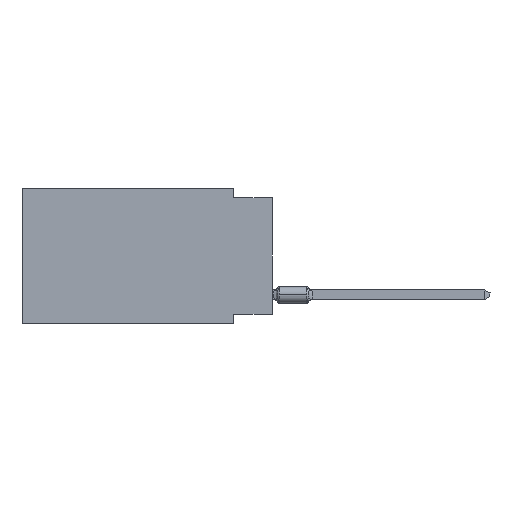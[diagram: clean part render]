
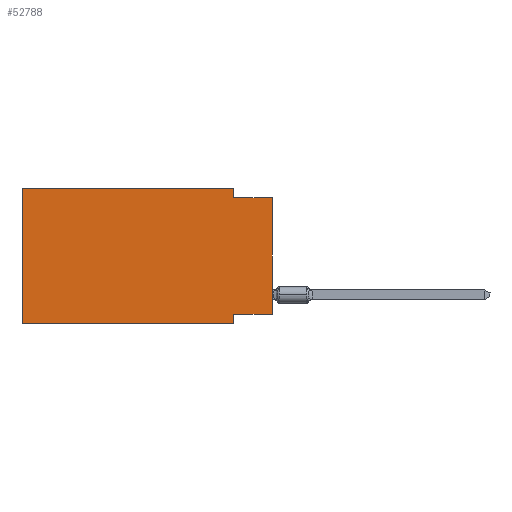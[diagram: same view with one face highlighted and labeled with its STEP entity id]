
A CAD part, left-side view. The second image highlights one B-rep face of the part: STEP entity #52788.
In plain terms, the highlighted planar face has unit normal (-1, 0, 0).
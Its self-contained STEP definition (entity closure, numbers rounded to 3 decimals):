
#1383 = DIRECTION ( 'NONE',  ( 0., -1., 0. ) ) ;
#1533 = ORIENTED_EDGE ( 'NONE', *, *, #18060, .F. ) ;
#2192 = VECTOR ( 'NONE', #11639, 1000. ) ;
#2943 = DIRECTION ( 'NONE',  ( 1., 0., 0. ) ) ;
#3807 = VECTOR ( 'NONE', #10989, 1000. ) ;
#5880 = CARTESIAN_POINT ( 'NONE',  ( 0., 2.54, 0. ) ) ;
#6173 = CARTESIAN_POINT ( 'NONE',  ( 0., 16.383, 0. ) ) ;
#8755 = LINE ( 'NONE', #69886, #24046 ) ;
#9847 = DIRECTION ( 'NONE',  ( 0., -1., 0. ) ) ;
#10810 = DIRECTION ( 'NONE',  ( 0., 0., -1. ) ) ;
#10989 = DIRECTION ( 'NONE',  ( 0., 1., 0. ) ) ;
#11277 = EDGE_CURVE ( 'NONE', #36131, #18457, #34651, .T. ) ;
#11639 = DIRECTION ( 'NONE',  ( 0., -1., 0. ) ) ;
#15030 = LINE ( 'NONE', #37718, #3807 ) ;
#15387 = EDGE_CURVE ( 'NONE', #43830, #36131, #8755, .T. ) ;
#15999 = VERTEX_POINT ( 'NONE', #23477 ) ;
#18060 = EDGE_CURVE ( 'NONE', #28030, #43830, #68750, .T. ) ;
#18457 = VERTEX_POINT ( 'NONE', #68885 ) ;
#18675 = EDGE_LOOP ( 'NONE', ( #70480, #69194, #62067, #1533, #72188, #52999, #63811, #28045 ) ) ;
#19309 = VECTOR ( 'NONE', #9847, 1000. ) ;
#19745 = CARTESIAN_POINT ( 'NONE',  ( 0., 16.383, 0. ) ) ;
#20841 = VERTEX_POINT ( 'NONE', #34207 ) ;
#22813 = EDGE_CURVE ( 'NONE', #15999, #20841, #15030, .T. ) ;
#23095 = CARTESIAN_POINT ( 'NONE',  ( 0., 0., 0. ) ) ;
#23446 = LINE ( 'NONE', #23095, #54664 ) ;
#23477 = CARTESIAN_POINT ( 'NONE',  ( 0., 0., -8.255 ) ) ;
#24046 = VECTOR ( 'NONE', #24820, 1000. ) ;
#24353 = VECTOR ( 'NONE', #10810, 1000. ) ;
#24820 = DIRECTION ( 'NONE',  ( 0., 0., -1. ) ) ;
#24863 = DIRECTION ( 'NONE',  ( 0., 0., -1. ) ) ;
#28030 = VERTEX_POINT ( 'NONE', #56153 ) ;
#28045 = ORIENTED_EDGE ( 'NONE', *, *, #22813, .F. ) ;
#28693 = CARTESIAN_POINT ( 'NONE',  ( 0., 2.54, -0.635 ) ) ;
#31381 = CARTESIAN_POINT ( 'NONE',  ( 0., 16.383, 0. ) ) ;
#32398 = CARTESIAN_POINT ( 'NONE',  ( 0., 2.54, -8.89 ) ) ;
#34207 = CARTESIAN_POINT ( 'NONE',  ( 0., 2.54, -8.255 ) ) ;
#34354 = VECTOR ( 'NONE', #52305, 1000. ) ;
#34651 = LINE ( 'NONE', #39442, #43496 ) ;
#36131 = VERTEX_POINT ( 'NONE', #28693 ) ;
#36876 = LINE ( 'NONE', #31381, #34354 ) ;
#37718 = CARTESIAN_POINT ( 'NONE',  ( 0., 0., -8.255 ) ) ;
#39442 = CARTESIAN_POINT ( 'NONE',  ( 0., 0., -0.635 ) ) ;
#39960 = DIRECTION ( 'NONE',  ( 0., 0., 1. ) ) ;
#40464 = EDGE_CURVE ( 'NONE', #45413, #28030, #36876, .T. ) ;
#43496 = VECTOR ( 'NONE', #1383, 1000. ) ;
#43830 = VERTEX_POINT ( 'NONE', #5880 ) ;
#43867 = LINE ( 'NONE', #60739, #19309 ) ;
#44091 = EDGE_CURVE ( 'NONE', #20841, #55934, #54048, .T. ) ;
#45413 = VERTEX_POINT ( 'NONE', #51855 ) ;
#48443 = AXIS2_PLACEMENT_3D ( 'NONE', #19745, #2943, #24863 ) ;
#51855 = CARTESIAN_POINT ( 'NONE',  ( 0., 16.383, -8.89 ) ) ;
#52305 = DIRECTION ( 'NONE',  ( 0., 0., 1. ) ) ;
#52736 = FACE_OUTER_BOUND ( 'NONE', #18675, .T. ) ;
#52788 = ADVANCED_FACE ( 'NONE', ( #52736 ), #69562, .F. ) ;
#52999 = ORIENTED_EDGE ( 'NONE', *, *, #53701, .T. ) ;
#53701 = EDGE_CURVE ( 'NONE', #45413, #55934, #43867, .T. ) ;
#54048 = LINE ( 'NONE', #32398, #24353 ) ;
#54664 = VECTOR ( 'NONE', #39960, 1000. ) ;
#55934 = VERTEX_POINT ( 'NONE', #63453 ) ;
#56153 = CARTESIAN_POINT ( 'NONE',  ( 0., 16.383, 0. ) ) ;
#57375 = EDGE_CURVE ( 'NONE', #15999, #18457, #23446, .T. ) ;
#60739 = CARTESIAN_POINT ( 'NONE',  ( 0., 16.383, -8.89 ) ) ;
#62067 = ORIENTED_EDGE ( 'NONE', *, *, #15387, .F. ) ;
#63453 = CARTESIAN_POINT ( 'NONE',  ( 0., 2.54, -8.89 ) ) ;
#63811 = ORIENTED_EDGE ( 'NONE', *, *, #44091, .F. ) ;
#68750 = LINE ( 'NONE', #6173, #2192 ) ;
#68885 = CARTESIAN_POINT ( 'NONE',  ( 0., 0., -0.635 ) ) ;
#69194 = ORIENTED_EDGE ( 'NONE', *, *, #11277, .F. ) ;
#69562 = PLANE ( 'NONE',  #48443 ) ;
#69886 = CARTESIAN_POINT ( 'NONE',  ( 0., 2.54, 0. ) ) ;
#70480 = ORIENTED_EDGE ( 'NONE', *, *, #57375, .T. ) ;
#72188 = ORIENTED_EDGE ( 'NONE', *, *, #40464, .F. ) ;
